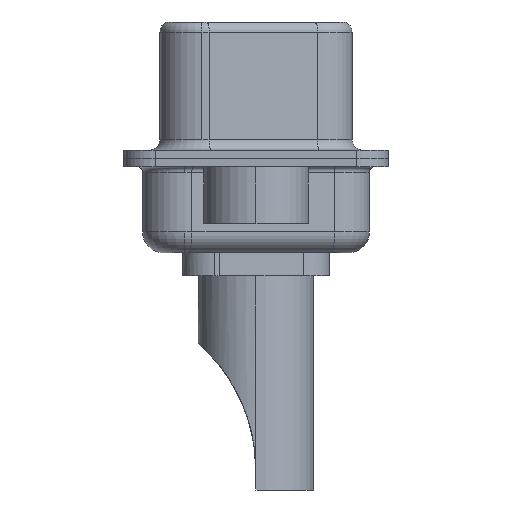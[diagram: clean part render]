
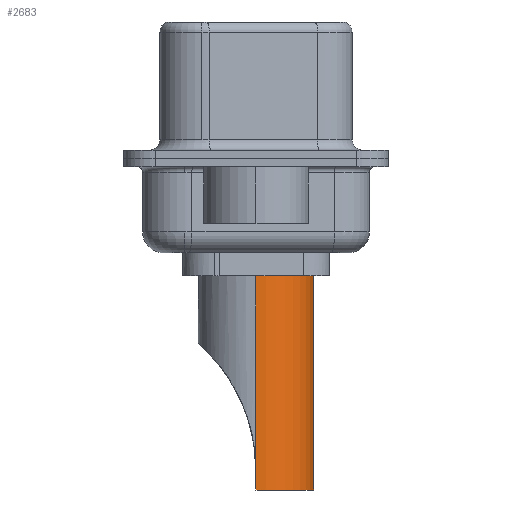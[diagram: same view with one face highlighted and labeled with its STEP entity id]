
A CAD part, left-side view. The second image highlights one B-rep face of the part: STEP entity #2683.
In plain terms, the highlighted cylindrical face has radius 2.75 mm (diameter 5.5 mm), a partial arc.
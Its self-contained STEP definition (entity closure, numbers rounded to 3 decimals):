
#203 = VERTEX_POINT ( 'NONE', #11921 ) ;
#706 = VECTOR ( 'NONE', #10720, 1000. ) ;
#1313 = ORIENTED_EDGE ( 'NONE', *, *, #21059, .F. ) ;
#1606 = DIRECTION ( 'NONE',  ( 0., 0., 1. ) ) ;
#1783 = EDGE_CURVE ( 'NONE', #203, #9671, #15610, .T. ) ;
#1987 = CARTESIAN_POINT ( 'NONE',  ( 0., 0., 1.5 ) ) ;
#2617 = CIRCLE ( 'NONE', #4395, 2.75 ) ;
#2683 = ADVANCED_FACE ( 'NONE', ( #8218 ), #18598, .T. ) ;
#3536 = CIRCLE ( 'NONE', #8829, 2.75 ) ;
#4052 = DIRECTION ( 'NONE',  ( 0., 0., -1. ) ) ;
#4395 = AXIS2_PLACEMENT_3D ( 'NONE', #19041, #1606, #13476 ) ;
#4606 = CARTESIAN_POINT ( 'NONE',  ( 2.75, 0., -8.7 ) ) ;
#4731 = DIRECTION ( 'NONE',  ( 0., 0., 1. ) ) ;
#5621 = CARTESIAN_POINT ( 'NONE',  ( 2.75, 0., -8.7 ) ) ;
#5666 = VECTOR ( 'NONE', #17574, 1000. ) ;
#6695 = LINE ( 'NONE', #8520, #706 ) ;
#6860 = ORIENTED_EDGE ( 'NONE', *, *, #8083, .F. ) ;
#7249 = DIRECTION ( 'NONE',  ( 1., 0., 0. ) ) ;
#7552 = EDGE_CURVE ( 'NONE', #18118, #8049, #15481, .T. ) ;
#8049 = VERTEX_POINT ( 'NONE', #21137 ) ;
#8083 = EDGE_CURVE ( 'NONE', #18118, #13683, #11121, .T. ) ;
#8218 = FACE_OUTER_BOUND ( 'NONE', #22370, .T. ) ;
#8520 = CARTESIAN_POINT ( 'NONE',  ( 2.75, 0., 4.234 ) ) ;
#8829 = AXIS2_PLACEMENT_3D ( 'NONE', #1987, #4731, #17879 ) ;
#9671 = VERTEX_POINT ( 'NONE', #4606 ) ;
#9904 = EDGE_CURVE ( 'NONE', #8049, #9671, #2617, .T. ) ;
#10304 = ORIENTED_EDGE ( 'NONE', *, *, #10380, .T. ) ;
#10380 = EDGE_CURVE ( 'NONE', #203, #15868, #6695, .T. ) ;
#10720 = DIRECTION ( 'NONE',  ( 0., 0., 1. ) ) ;
#10820 = CARTESIAN_POINT ( 'NONE',  ( -2.75, 0., -8.7 ) ) ;
#11121 = LINE ( 'NONE', #14146, #5666 ) ;
#11261 = AXIS2_PLACEMENT_3D ( 'NONE', #15762, #17652, #7249 ) ;
#11508 = VECTOR ( 'NONE', #4052, 1000. ) ;
#11921 = CARTESIAN_POINT ( 'NONE',  ( 2.75, 0., -7.764 ) ) ;
#12260 = ORIENTED_EDGE ( 'NONE', *, *, #1783, .F. ) ;
#12762 = VECTOR ( 'NONE', #21432, 1000. ) ;
#12850 = ORIENTED_EDGE ( 'NONE', *, *, #9904, .T. ) ;
#12941 = ORIENTED_EDGE ( 'NONE', *, *, #7552, .T. ) ;
#13476 = DIRECTION ( 'NONE',  ( 1., 0., 0. ) ) ;
#13683 = VERTEX_POINT ( 'NONE', #17184 ) ;
#14146 = CARTESIAN_POINT ( 'NONE',  ( -2.75, 0., 4.234 ) ) ;
#15257 = CARTESIAN_POINT ( 'NONE',  ( 2.75, 0., 1.5 ) ) ;
#15481 = LINE ( 'NONE', #10820, #12762 ) ;
#15610 = LINE ( 'NONE', #5621, #11508 ) ;
#15762 = CARTESIAN_POINT ( 'NONE',  ( 0., 0., 4.234 ) ) ;
#15868 = VERTEX_POINT ( 'NONE', #15257 ) ;
#17184 = CARTESIAN_POINT ( 'NONE',  ( -2.75, 0., 1.5 ) ) ;
#17574 = DIRECTION ( 'NONE',  ( 0., 0., 1. ) ) ;
#17652 = DIRECTION ( 'NONE',  ( 0., 0., 1. ) ) ;
#17879 = DIRECTION ( 'NONE',  ( 1., 0., 0. ) ) ;
#18118 = VERTEX_POINT ( 'NONE', #19727 ) ;
#18598 = CYLINDRICAL_SURFACE ( 'NONE', #11261, 2.75 ) ;
#19041 = CARTESIAN_POINT ( 'NONE',  ( 0., 0., -8.7 ) ) ;
#19727 = CARTESIAN_POINT ( 'NONE',  ( -2.75, 0., -7.764 ) ) ;
#21059 = EDGE_CURVE ( 'NONE', #13683, #15868, #3536, .T. ) ;
#21137 = CARTESIAN_POINT ( 'NONE',  ( -2.75, 0., -8.7 ) ) ;
#21432 = DIRECTION ( 'NONE',  ( 0., 0., -1. ) ) ;
#22370 = EDGE_LOOP ( 'NONE', ( #6860, #12941, #12850, #12260, #10304, #1313 ) ) ;
